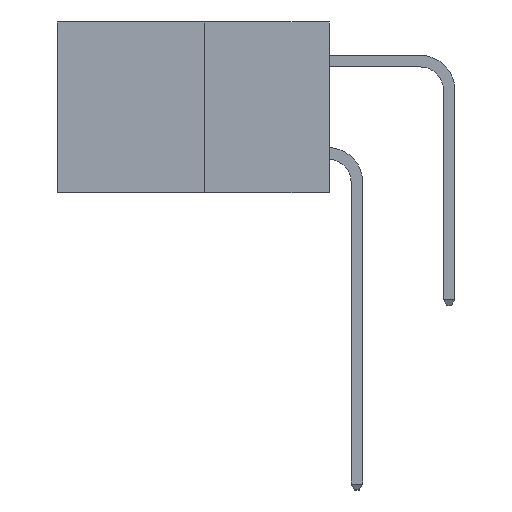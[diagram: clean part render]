
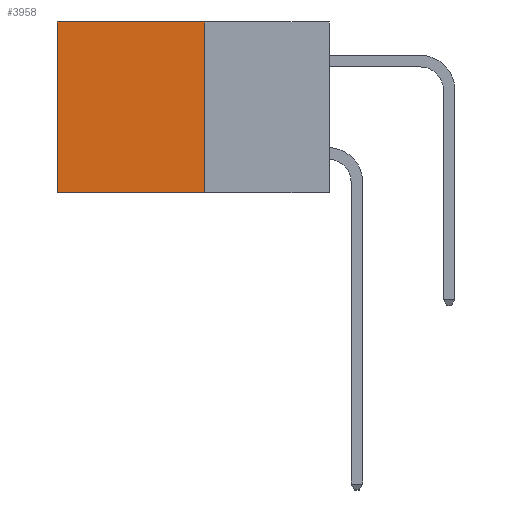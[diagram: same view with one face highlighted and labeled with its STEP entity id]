
A CAD part, left-side view. The second image highlights one B-rep face of the part: STEP entity #3958.
In plain terms, the highlighted planar face has unit normal (-1, 0, 0).
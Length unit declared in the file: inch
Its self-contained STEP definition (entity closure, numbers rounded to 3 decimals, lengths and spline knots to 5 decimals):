
#435 = DIRECTION ( 'NONE',  ( 0., 0., -1. ) ) ;
#551 = FACE_OUTER_BOUND ( 'NONE', #13235, .T. ) ;
#963 = LINE ( 'NONE', #7137, #7594 ) ;
#1761 = CARTESIAN_POINT ( 'NONE',  ( 0.277, 0.27, -0.37 ) ) ;
#3164 = VERTEX_POINT ( 'NONE', #13159 ) ;
#3354 = EDGE_CURVE ( 'NONE', #3164, #11694, #10780, .T. ) ;
#3804 = VECTOR ( 'NONE', #8357, 39.37008 ) ;
#3958 = ADVANCED_FACE ( 'NONE', ( #551 ), #14550, .F. ) ;
#4417 = CARTESIAN_POINT ( 'NONE',  ( 0.277, 0.59, 0. ) ) ;
#5135 = VECTOR ( 'NONE', #14800, 39.37008 ) ;
#6234 = EDGE_CURVE ( 'NONE', #9062, #11694, #963, .T. ) ;
#6763 = CARTESIAN_POINT ( 'NONE',  ( 0.277, 0.27, -0.37 ) ) ;
#6838 = EDGE_CURVE ( 'NONE', #11990, #3164, #8596, .T. ) ;
#7137 = CARTESIAN_POINT ( 'NONE',  ( 0.277, 0.59, -0.37 ) ) ;
#7594 = VECTOR ( 'NONE', #435, 39.37008 ) ;
#7679 = ORIENTED_EDGE ( 'NONE', *, *, #11976, .T. ) ;
#8069 = DIRECTION ( 'NONE',  ( 0., 0., -1. ) ) ;
#8357 = DIRECTION ( 'NONE',  ( 0., 1., 0. ) ) ;
#8497 = CARTESIAN_POINT ( 'NONE',  ( 0.277, 0.27, 0. ) ) ;
#8596 = LINE ( 'NONE', #10910, #5135 ) ;
#9062 = VERTEX_POINT ( 'NONE', #4417 ) ;
#9152 = CARTESIAN_POINT ( 'NONE',  ( 0.277, 0.59, -0.37 ) ) ;
#9731 = ORIENTED_EDGE ( 'NONE', *, *, #6838, .F. ) ;
#10780 = LINE ( 'NONE', #1761, #3804 ) ;
#10910 = CARTESIAN_POINT ( 'NONE',  ( 0.277, 0.27, -0.37 ) ) ;
#11694 = VERTEX_POINT ( 'NONE', #9152 ) ;
#11851 = ORIENTED_EDGE ( 'NONE', *, *, #6234, .T. ) ;
#11976 = EDGE_CURVE ( 'NONE', #11990, #9062, #16041, .T. ) ;
#11990 = VERTEX_POINT ( 'NONE', #8497 ) ;
#12533 = ORIENTED_EDGE ( 'NONE', *, *, #3354, .F. ) ;
#12615 = VECTOR ( 'NONE', #16245, 39.37008 ) ;
#13159 = CARTESIAN_POINT ( 'NONE',  ( 0.277, 0.27, -0.37 ) ) ;
#13235 = EDGE_LOOP ( 'NONE', ( #11851, #12533, #9731, #7679 ) ) ;
#14550 = PLANE ( 'NONE',  #16685 ) ;
#14800 = DIRECTION ( 'NONE',  ( 0., 0., -1. ) ) ;
#15852 = DIRECTION ( 'NONE',  ( 1., 0., 0. ) ) ;
#16041 = LINE ( 'NONE', #16191, #12615 ) ;
#16191 = CARTESIAN_POINT ( 'NONE',  ( 0.277, 0.27, 0. ) ) ;
#16245 = DIRECTION ( 'NONE',  ( 0., 1., 0. ) ) ;
#16685 = AXIS2_PLACEMENT_3D ( 'NONE', #6763, #15852, #8069 ) ;
